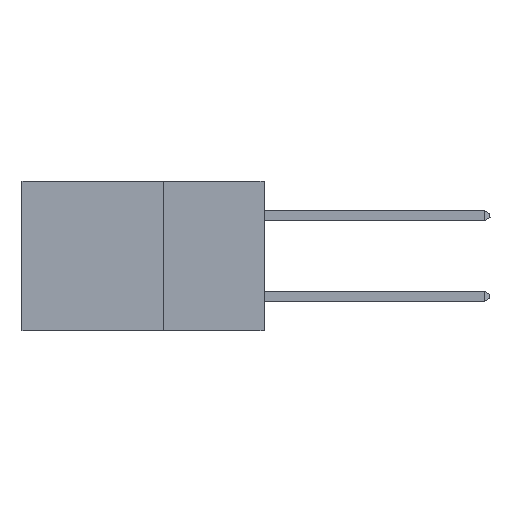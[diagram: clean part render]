
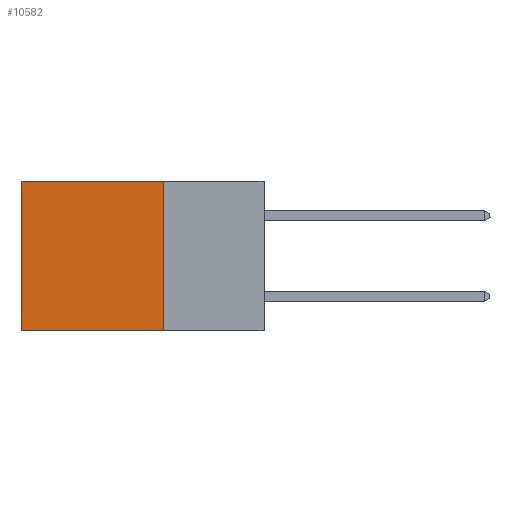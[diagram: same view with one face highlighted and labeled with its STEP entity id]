
A CAD part, left-side view. The second image highlights one B-rep face of the part: STEP entity #10582.
In plain terms, the highlighted planar face has unit normal (-1, 0, 0).
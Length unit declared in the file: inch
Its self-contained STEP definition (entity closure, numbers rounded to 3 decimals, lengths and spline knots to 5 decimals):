
#813 = ORIENTED_EDGE ( 'NONE', *, *, #13655, .F. ) ;
#2322 = EDGE_CURVE ( 'NONE', #17636, #9802, #7012, .T. ) ;
#3227 = LINE ( 'NONE', #9993, #7071 ) ;
#3505 = EDGE_CURVE ( 'NONE', #10038, #9802, #14955, .T. ) ;
#4803 = CARTESIAN_POINT ( 'NONE',  ( 0.298, 0.25, -0.37 ) ) ;
#7012 = LINE ( 'NONE', #21456, #19159 ) ;
#7071 = VECTOR ( 'NONE', #25786, 39.37008 ) ;
#8047 = VECTOR ( 'NONE', #10834, 39.37008 ) ;
#9074 = CARTESIAN_POINT ( 'NONE',  ( 0.298, 0.6, -0.37 ) ) ;
#9623 = EDGE_CURVE ( 'NONE', #15851, #10038, #3227, .T. ) ;
#9802 = VERTEX_POINT ( 'NONE', #9074 ) ;
#9993 = CARTESIAN_POINT ( 'NONE',  ( 0.298, 0.25, 0. ) ) ;
#10038 = VERTEX_POINT ( 'NONE', #18958 ) ;
#10273 = EDGE_LOOP ( 'NONE', ( #19735, #21171, #813, #20951 ) ) ;
#10582 = ADVANCED_FACE ( 'NONE', ( #19539 ), #25170, .F. ) ;
#10820 = CARTESIAN_POINT ( 'NONE',  ( 0.298, 0.25, 0. ) ) ;
#10834 = DIRECTION ( 'NONE',  ( 0., 0., -1. ) ) ;
#13655 = EDGE_CURVE ( 'NONE', #15851, #17636, #19831, .T. ) ;
#14235 = DIRECTION ( 'NONE',  ( 0., 0., -1. ) ) ;
#14955 = LINE ( 'NONE', #17702, #8047 ) ;
#15851 = VERTEX_POINT ( 'NONE', #27919 ) ;
#16246 = AXIS2_PLACEMENT_3D ( 'NONE', #18492, #22844, #14235 ) ;
#17636 = VERTEX_POINT ( 'NONE', #4803 ) ;
#17702 = CARTESIAN_POINT ( 'NONE',  ( 0.298, 0.6, 0. ) ) ;
#18492 = CARTESIAN_POINT ( 'NONE',  ( 0.298, 0.25, 0. ) ) ;
#18958 = CARTESIAN_POINT ( 'NONE',  ( 0.298, 0.6, 0. ) ) ;
#19159 = VECTOR ( 'NONE', #28129, 39.37008 ) ;
#19539 = FACE_OUTER_BOUND ( 'NONE', #10273, .T. ) ;
#19735 = ORIENTED_EDGE ( 'NONE', *, *, #3505, .T. ) ;
#19831 = LINE ( 'NONE', #10820, #21204 ) ;
#20951 = ORIENTED_EDGE ( 'NONE', *, *, #9623, .T. ) ;
#21171 = ORIENTED_EDGE ( 'NONE', *, *, #2322, .F. ) ;
#21204 = VECTOR ( 'NONE', #26614, 39.37008 ) ;
#21456 = CARTESIAN_POINT ( 'NONE',  ( 0.298, 0.25, -0.37 ) ) ;
#22844 = DIRECTION ( 'NONE',  ( 1., 0., 0. ) ) ;
#25170 = PLANE ( 'NONE',  #16246 ) ;
#25786 = DIRECTION ( 'NONE',  ( 0., 1., 0. ) ) ;
#26614 = DIRECTION ( 'NONE',  ( 0., 0., -1. ) ) ;
#27919 = CARTESIAN_POINT ( 'NONE',  ( 0.298, 0.25, 0. ) ) ;
#28129 = DIRECTION ( 'NONE',  ( 0., 1., 0. ) ) ;
